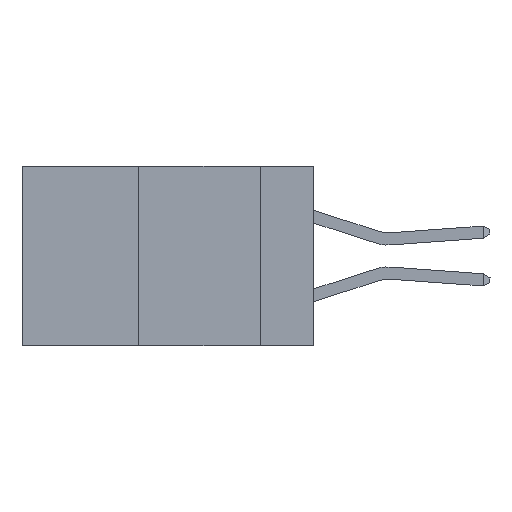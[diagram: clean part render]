
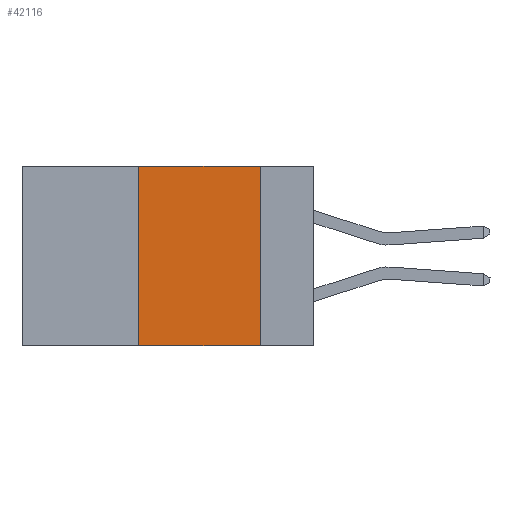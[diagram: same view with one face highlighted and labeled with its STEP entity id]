
A CAD part, left-side view. The second image highlights one B-rep face of the part: STEP entity #42116.
In plain terms, the highlighted planar face has unit normal (-1, 0, 0).
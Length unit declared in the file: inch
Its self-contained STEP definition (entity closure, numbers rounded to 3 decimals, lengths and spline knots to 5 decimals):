
#991 = DIRECTION ( 'NONE',  ( 1., 0., 0. ) ) ;
#2601 = LINE ( 'NONE', #34166, #29834 ) ;
#4112 = CARTESIAN_POINT ( 'NONE',  ( 0., 0.36, 0. ) ) ;
#4278 = PLANE ( 'NONE',  #18322 ) ;
#5743 = ORIENTED_EDGE ( 'NONE', *, *, #37434, .F. ) ;
#6121 = DIRECTION ( 'NONE',  ( 0., -1., 0. ) ) ;
#9803 = ORIENTED_EDGE ( 'NONE', *, *, #10290, .F. ) ;
#10290 = EDGE_CURVE ( 'NONE', #30033, #19875, #39127, .T. ) ;
#10933 = VECTOR ( 'NONE', #24560, 39.37008 ) ;
#11843 = VECTOR ( 'NONE', #6121, 39.37008 ) ;
#13674 = DIRECTION ( 'NONE',  ( 0., -1., 0. ) ) ;
#13731 = FACE_OUTER_BOUND ( 'NONE', #38589, .T. ) ;
#15293 = ORIENTED_EDGE ( 'NONE', *, *, #29204, .T. ) ;
#17879 = VERTEX_POINT ( 'NONE', #19313 ) ;
#18222 = LINE ( 'NONE', #20988, #27291 ) ;
#18322 = AXIS2_PLACEMENT_3D ( 'NONE', #21431, #991, #24865 ) ;
#19313 = CARTESIAN_POINT ( 'NONE',  ( 0., 0.11, -0.37 ) ) ;
#19875 = VERTEX_POINT ( 'NONE', #25871 ) ;
#20988 = CARTESIAN_POINT ( 'NONE',  ( 0., 0.11, 0. ) ) ;
#21431 = CARTESIAN_POINT ( 'NONE',  ( 0., 0.6, 0. ) ) ;
#23146 = CARTESIAN_POINT ( 'NONE',  ( 0., 0.6, 0. ) ) ;
#24560 = DIRECTION ( 'NONE',  ( 0., 0., 1. ) ) ;
#24865 = DIRECTION ( 'NONE',  ( 0., 0., -1. ) ) ;
#25871 = CARTESIAN_POINT ( 'NONE',  ( 0., 0.11, 0. ) ) ;
#27291 = VECTOR ( 'NONE', #41462, 39.37008 ) ;
#29204 = EDGE_CURVE ( 'NONE', #34026, #17879, #2601, .T. ) ;
#29834 = VECTOR ( 'NONE', #13674, 39.37008 ) ;
#30033 = VERTEX_POINT ( 'NONE', #40083 ) ;
#30191 = LINE ( 'NONE', #4112, #10933 ) ;
#31552 = EDGE_CURVE ( 'NONE', #34026, #30033, #30191, .T. ) ;
#34026 = VERTEX_POINT ( 'NONE', #35950 ) ;
#34166 = CARTESIAN_POINT ( 'NONE',  ( 0., 0.6, -0.37 ) ) ;
#35950 = CARTESIAN_POINT ( 'NONE',  ( 0., 0.36, -0.37 ) ) ;
#37434 = EDGE_CURVE ( 'NONE', #19875, #17879, #18222, .T. ) ;
#38589 = EDGE_LOOP ( 'NONE', ( #5743, #9803, #43179, #15293 ) ) ;
#39127 = LINE ( 'NONE', #23146, #11843 ) ;
#40083 = CARTESIAN_POINT ( 'NONE',  ( 0., 0.36, 0. ) ) ;
#41462 = DIRECTION ( 'NONE',  ( 0., 0., -1. ) ) ;
#42116 = ADVANCED_FACE ( 'NONE', ( #13731 ), #4278, .F. ) ;
#43179 = ORIENTED_EDGE ( 'NONE', *, *, #31552, .F. ) ;
